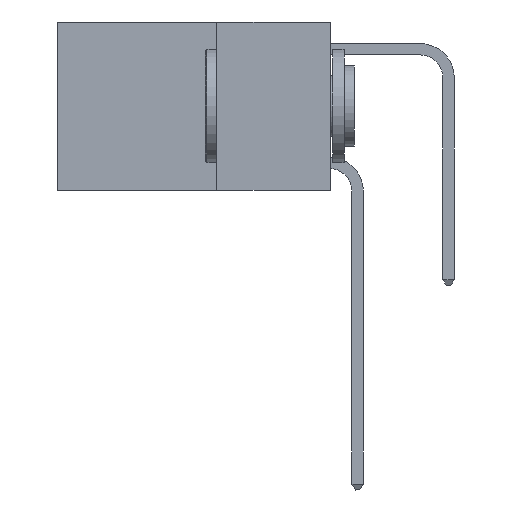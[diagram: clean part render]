
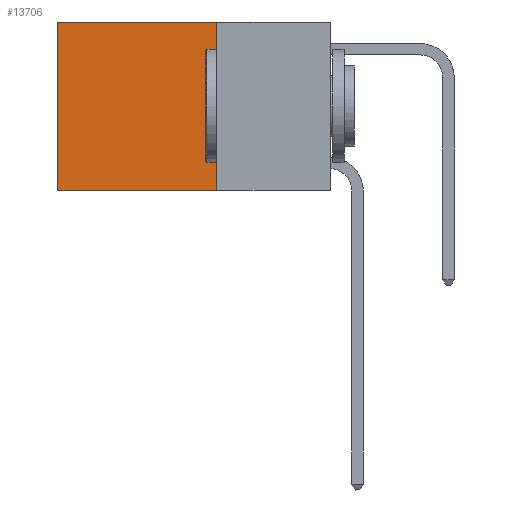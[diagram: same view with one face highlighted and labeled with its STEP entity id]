
A CAD part, left-side view. The second image highlights one B-rep face of the part: STEP entity #13706.
In plain terms, the highlighted planar face has unit normal (-1, 0, 0).
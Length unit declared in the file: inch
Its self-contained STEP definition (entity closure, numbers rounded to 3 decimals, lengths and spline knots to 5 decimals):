
#1550 = CARTESIAN_POINT ( 'NONE',  ( 0.2625, 0.25, 0. ) ) ;
#1730 = ORIENTED_EDGE ( 'NONE', *, *, #21107, .F. ) ;
#1882 = ORIENTED_EDGE ( 'NONE', *, *, #22809, .T. ) ;
#2292 = EDGE_CURVE ( 'NONE', #29534, #12801, #26815, .T. ) ;
#4792 = DIRECTION ( 'NONE',  ( 0., 1., 0. ) ) ;
#6370 = CARTESIAN_POINT ( 'NONE',  ( 0.2625, 0.25, 0. ) ) ;
#6397 = VECTOR ( 'NONE', #6709, 39.37008 ) ;
#6709 = DIRECTION ( 'NONE',  ( 0., 0., -1. ) ) ;
#6932 = ORIENTED_EDGE ( 'NONE', *, *, #22200, .F. ) ;
#7637 = PLANE ( 'NONE',  #14907 ) ;
#8229 = CARTESIAN_POINT ( 'NONE',  ( 0.2625, 0.25, 0. ) ) ;
#8254 = VERTEX_POINT ( 'NONE', #8229 ) ;
#9322 = CARTESIAN_POINT ( 'NONE',  ( 0.2625, 0.6, -0.37 ) ) ;
#9513 = CARTESIAN_POINT ( 'NONE',  ( 0.2625, 0.6, 0. ) ) ;
#10011 = VERTEX_POINT ( 'NONE', #14543 ) ;
#12640 = DIRECTION ( 'NONE',  ( 1., 0., 0. ) ) ;
#12801 = VERTEX_POINT ( 'NONE', #9322 ) ;
#13390 = VECTOR ( 'NONE', #28701, 39.37008 ) ;
#13405 = FACE_OUTER_BOUND ( 'NONE', #18002, .T. ) ;
#13706 = ADVANCED_FACE ( 'NONE', ( #13405 ), #7637, .F. ) ;
#14510 = LINE ( 'NONE', #6370, #26780 ) ;
#14543 = CARTESIAN_POINT ( 'NONE',  ( 0.2625, 0.25, -0.37 ) ) ;
#14907 = AXIS2_PLACEMENT_3D ( 'NONE', #15022, #12640, #29806 ) ;
#15022 = CARTESIAN_POINT ( 'NONE',  ( 0.2625, 0.25, 0. ) ) ;
#18002 = EDGE_LOOP ( 'NONE', ( #29167, #1730, #6932, #1882 ) ) ;
#19002 = CARTESIAN_POINT ( 'NONE',  ( 0.2625, 0.6, 0. ) ) ;
#21107 = EDGE_CURVE ( 'NONE', #10011, #12801, #31090, .T. ) ;
#22200 = EDGE_CURVE ( 'NONE', #8254, #10011, #31387, .T. ) ;
#22809 = EDGE_CURVE ( 'NONE', #8254, #29534, #14510, .T. ) ;
#26070 = DIRECTION ( 'NONE',  ( 0., 1., 0. ) ) ;
#26780 = VECTOR ( 'NONE', #26070, 39.37008 ) ;
#26815 = LINE ( 'NONE', #19002, #6397 ) ;
#28701 = DIRECTION ( 'NONE',  ( 0., 0., -1. ) ) ;
#29167 = ORIENTED_EDGE ( 'NONE', *, *, #2292, .T. ) ;
#29534 = VERTEX_POINT ( 'NONE', #9513 ) ;
#29806 = DIRECTION ( 'NONE',  ( 0., 0., -1. ) ) ;
#31090 = LINE ( 'NONE', #31898, #31831 ) ;
#31387 = LINE ( 'NONE', #1550, #13390 ) ;
#31831 = VECTOR ( 'NONE', #4792, 39.37008 ) ;
#31898 = CARTESIAN_POINT ( 'NONE',  ( 0.2625, 0.25, -0.37 ) ) ;
